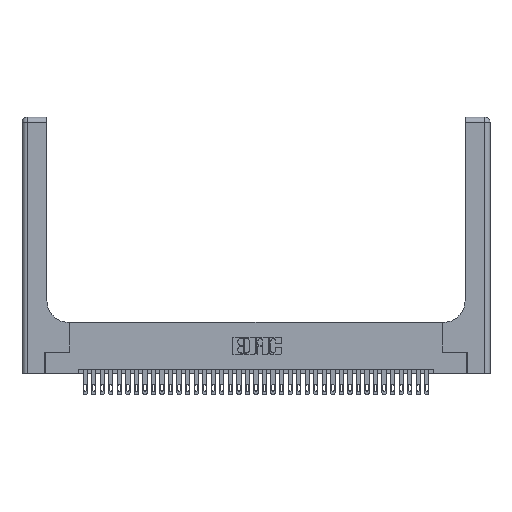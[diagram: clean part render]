
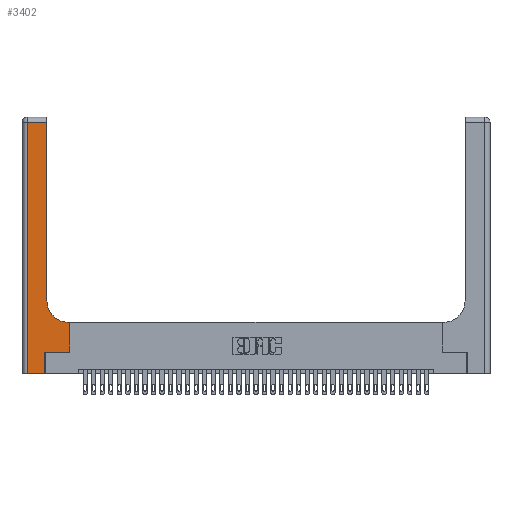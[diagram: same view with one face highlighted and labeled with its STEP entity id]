
A CAD part, top view. The second image highlights one B-rep face of the part: STEP entity #3402.
In plain terms, the highlighted planar face has unit normal (0, 0, 1).
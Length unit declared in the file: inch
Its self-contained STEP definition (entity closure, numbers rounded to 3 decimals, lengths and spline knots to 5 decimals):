
#391 = DIRECTION ( 'NONE',  ( -1., 0., 0. ) ) ;
#893 = VECTOR ( 'NONE', #2784, 39.37008 ) ;
#1123 = VERTEX_POINT ( 'NONE', #20620 ) ;
#1534 = DIRECTION ( 'NONE',  ( 0., -1., 0. ) ) ;
#1537 = CARTESIAN_POINT ( 'NONE',  ( 0.269, 0., 0.37 ) ) ;
#1627 = VERTEX_POINT ( 'NONE', #18976 ) ;
#2714 = EDGE_CURVE ( 'NONE', #26337, #1627, #14460, .T. ) ;
#2784 = DIRECTION ( 'NONE',  ( 0., 1., 0. ) ) ;
#3259 = CARTESIAN_POINT ( 'NONE',  ( 0.06, 2.94, 0.37 ) ) ;
#3286 = LINE ( 'NONE', #9395, #13718 ) ;
#3402 = ADVANCED_FACE ( 'NONE', ( #23011 ), #7771, .F. ) ;
#3917 = CARTESIAN_POINT ( 'NONE',  ( 0.2915, 3., 0.37 ) ) ;
#4091 = CARTESIAN_POINT ( 'NONE',  ( 0.06, 3., 0.37 ) ) ;
#4257 = CARTESIAN_POINT ( 'NONE',  ( 0.2915, 0.85, 0.37 ) ) ;
#4454 = DIRECTION ( 'NONE',  ( 0., 1., 0. ) ) ;
#4481 = VECTOR ( 'NONE', #19284, 39.37008 ) ;
#4587 = VERTEX_POINT ( 'NONE', #3259 ) ;
#5018 = ORIENTED_EDGE ( 'NONE', *, *, #21720, .T. ) ;
#6539 = CARTESIAN_POINT ( 'NONE',  ( 0.2915, 0.6, 0.37 ) ) ;
#6954 = DIRECTION ( 'NONE',  ( 1., 0., 0. ) ) ;
#7072 = VERTEX_POINT ( 'NONE', #4257 ) ;
#7271 = EDGE_CURVE ( 'NONE', #23634, #15143, #23150, .T. ) ;
#7636 = EDGE_CURVE ( 'NONE', #15143, #7072, #34808, .T. ) ;
#7721 = LINE ( 'NONE', #4091, #9049 ) ;
#7771 = PLANE ( 'NONE',  #34107 ) ;
#9049 = VECTOR ( 'NONE', #1534, 39.37008 ) ;
#9395 = CARTESIAN_POINT ( 'NONE',  ( 0., 0., 0.37 ) ) ;
#10273 = DIRECTION ( 'NONE',  ( 0., 1., 0. ) ) ;
#10623 = DIRECTION ( 'NONE',  ( -1., 0., 0. ) ) ;
#10814 = ORIENTED_EDGE ( 'NONE', *, *, #2714, .T. ) ;
#11134 = CARTESIAN_POINT ( 'NONE',  ( 0.269, 0.25, 0.37 ) ) ;
#11655 = ORIENTED_EDGE ( 'NONE', *, *, #16300, .T. ) ;
#11907 = EDGE_CURVE ( 'NONE', #33007, #26337, #27806, .T. ) ;
#12422 = ORIENTED_EDGE ( 'NONE', *, *, #7271, .T. ) ;
#13026 = CARTESIAN_POINT ( 'NONE',  ( 0.269, 0., 0.37 ) ) ;
#13184 = ORIENTED_EDGE ( 'NONE', *, *, #21218, .T. ) ;
#13547 = ORIENTED_EDGE ( 'NONE', *, *, #11907, .T. ) ;
#13718 = VECTOR ( 'NONE', #6954, 39.37008 ) ;
#13928 = VERTEX_POINT ( 'NONE', #22673 ) ;
#14452 = CARTESIAN_POINT ( 'NONE',  ( 0.5585, 0.25, 0.37 ) ) ;
#14460 = LINE ( 'NONE', #11134, #4481 ) ;
#15143 = VERTEX_POINT ( 'NONE', #30185 ) ;
#15825 = ORIENTED_EDGE ( 'NONE', *, *, #7636, .T. ) ;
#16300 = EDGE_CURVE ( 'NONE', #1627, #23634, #25007, .T. ) ;
#16527 = EDGE_CURVE ( 'NONE', #13928, #33007, #3286, .T. ) ;
#17266 = VECTOR ( 'NONE', #35808, 39.37008 ) ;
#17642 = CARTESIAN_POINT ( 'NONE',  ( 0., 2.94, 0.37 ) ) ;
#18931 = CARTESIAN_POINT ( 'NONE',  ( 0.5585, 0.6, 0.37 ) ) ;
#18976 = CARTESIAN_POINT ( 'NONE',  ( 0.5585, 0.25, 0.37 ) ) ;
#19284 = DIRECTION ( 'NONE',  ( 1., 0., 0. ) ) ;
#19867 = CARTESIAN_POINT ( 'NONE',  ( 0.269, 0.25, 0.37 ) ) ;
#20152 = VECTOR ( 'NONE', #10273, 39.37008 ) ;
#20620 = CARTESIAN_POINT ( 'NONE',  ( 0.2915, 2.94, 0.37 ) ) ;
#21033 = CARTESIAN_POINT ( 'NONE',  ( 0.5415, 0.85, 0.37 ) ) ;
#21057 = ORIENTED_EDGE ( 'NONE', *, *, #36758, .T. ) ;
#21218 = EDGE_CURVE ( 'NONE', #1123, #4587, #34156, .T. ) ;
#21720 = EDGE_CURVE ( 'NONE', #7072, #1123, #24387, .T. ) ;
#22673 = CARTESIAN_POINT ( 'NONE',  ( 0.06, 0., 0.37 ) ) ;
#22859 = ORIENTED_EDGE ( 'NONE', *, *, #16527, .T. ) ;
#23011 = FACE_OUTER_BOUND ( 'NONE', #27824, .T. ) ;
#23150 = LINE ( 'NONE', #6539, #17266 ) ;
#23634 = VERTEX_POINT ( 'NONE', #18931 ) ;
#23942 = DIRECTION ( 'NONE',  ( 0., 0., -1. ) ) ;
#24387 = LINE ( 'NONE', #3917, #28047 ) ;
#24659 = VECTOR ( 'NONE', #391, 39.37008 ) ;
#25007 = LINE ( 'NONE', #14452, #893 ) ;
#26337 = VERTEX_POINT ( 'NONE', #19867 ) ;
#27806 = LINE ( 'NONE', #13026, #20152 ) ;
#27824 = EDGE_LOOP ( 'NONE', ( #5018, #13184, #21057, #22859, #13547, #10814, #11655, #12422, #15825 ) ) ;
#27912 = DIRECTION ( 'NONE',  ( 0., 0., -1. ) ) ;
#28047 = VECTOR ( 'NONE', #4454, 39.37008 ) ;
#28198 = CARTESIAN_POINT ( 'NONE',  ( 0., 3., 0.37 ) ) ;
#30185 = CARTESIAN_POINT ( 'NONE',  ( 0.5415, 0.6, 0.37 ) ) ;
#33007 = VERTEX_POINT ( 'NONE', #1537 ) ;
#34107 = AXIS2_PLACEMENT_3D ( 'NONE', #28198, #27912, #10623 ) ;
#34156 = LINE ( 'NONE', #17642, #24659 ) ;
#34808 = CIRCLE ( 'NONE', #35569, 0.25 ) ;
#35569 = AXIS2_PLACEMENT_3D ( 'NONE', #21033, #23942, #35640 ) ;
#35640 = DIRECTION ( 'NONE',  ( 1., 0., 0. ) ) ;
#35808 = DIRECTION ( 'NONE',  ( -1., 0., 0. ) ) ;
#36758 = EDGE_CURVE ( 'NONE', #4587, #13928, #7721, .T. ) ;
